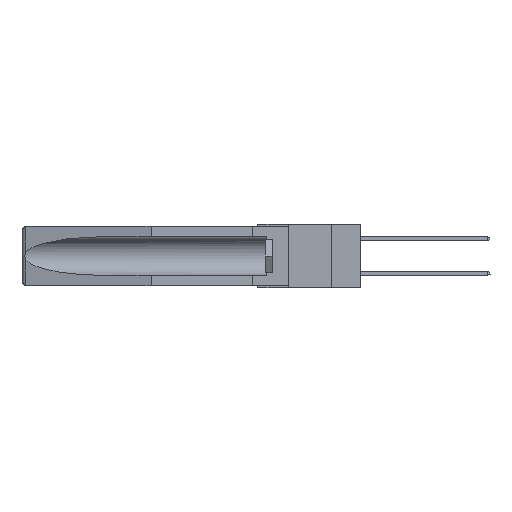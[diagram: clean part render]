
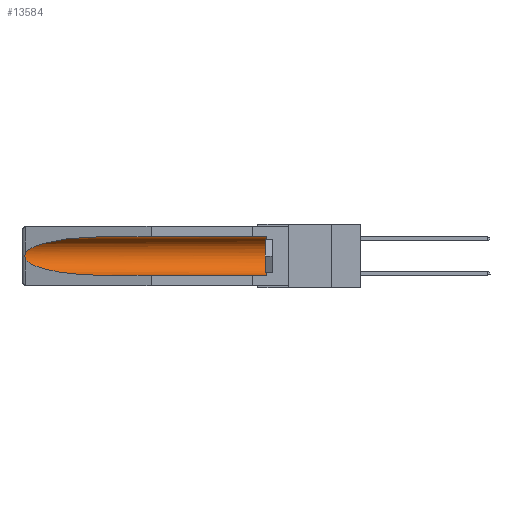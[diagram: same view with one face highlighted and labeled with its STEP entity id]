
A CAD part, left-side view. The second image highlights one B-rep face of the part: STEP entity #13584.
In plain terms, the highlighted cylindrical face has radius 2.857 mm (diameter 5.715 mm), a partial arc.
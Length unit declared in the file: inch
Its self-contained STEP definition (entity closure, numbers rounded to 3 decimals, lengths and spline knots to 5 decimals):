
#182 = CARTESIAN_POINT ( 'NONE',  ( 0.26537, 1.52718, -0.14972 ) ) ;
#677 =( BOUNDED_CURVE ( )  B_SPLINE_CURVE ( 3, ( #17258, #19397, #775, #2345 ),
 .UNSPECIFIED., .F., .F. ) 
 B_SPLINE_CURVE_WITH_KNOTS ( ( 4, 4 ),
 ( 0.1948, 1.5708 ),
 .UNSPECIFIED. ) 
 CURVE ( )  GEOMETRIC_REPRESENTATION_ITEM ( )  RATIONAL_B_SPLINE_CURVE ( ( 1., 0.848, 0.848, 1. ) ) 
 REPRESENTATION_ITEM ( '' )  );
#775 = CARTESIAN_POINT ( 'NONE',  ( 0.21114, 1.30732, -0.284 ) ) ;
#1628 = CARTESIAN_POINT ( 'NONE',  ( 0.25451, 1.48313, -0.09465 ) ) ;
#2092 = EDGE_CURVE ( 'NONE', #7967, #2964, #22281, .T. ) ;
#2345 = CARTESIAN_POINT ( 'NONE',  ( 0.155, 1.07973, -0.284 ) ) ;
#2677 = FACE_OUTER_BOUND ( 'NONE', #17705, .T. ) ;
#2744 = DIRECTION ( 'NONE',  ( 0., 1., 0. ) ) ;
#2804 = CARTESIAN_POINT ( 'NONE',  ( 0.26537, 1.52718, -0.19328 ) ) ;
#2964 = VERTEX_POINT ( 'NONE', #2804 ) ;
#3085 = AXIS2_PLACEMENT_3D ( 'NONE', #19926, #8956, #10681 ) ;
#3656 = CARTESIAN_POINT ( 'NONE',  ( 0.2673, 1.53269, -0.17917 ) ) ;
#3815 = CARTESIAN_POINT ( 'NONE',  ( 0.26654, 1.53092, -0.15636 ) ) ;
#3902 = CARTESIAN_POINT ( 'NONE',  ( 0.155, 1.07973, -0.059 ) ) ;
#3938 = EDGE_CURVE ( 'NONE', #17483, #12077, #10862, .T. ) ;
#4546 = CARTESIAN_POINT ( 'NONE',  ( 0.155, -0.30754, -0.059 ) ) ;
#6691 = VECTOR ( 'NONE', #20468, 39.37008 ) ;
#7471 = CARTESIAN_POINT ( 'NONE',  ( 0.155, -0.30754, -0.284 ) ) ;
#7504 = DIRECTION ( 'NONE',  ( 0., 0., 1. ) ) ;
#7678 = CYLINDRICAL_SURFACE ( 'NONE', #3085, 0.1125 ) ;
#7967 = VERTEX_POINT ( 'NONE', #19211 ) ;
#8046 = CARTESIAN_POINT ( 'NONE',  ( 0.155, 0.126, -0.059 ) ) ;
#8956 = DIRECTION ( 'NONE',  ( 0., 1., 0. ) ) ;
#9189 = CARTESIAN_POINT ( 'NONE',  ( 0.2675, 1.53308, -0.17534 ) ) ;
#9424 = VERTEX_POINT ( 'NONE', #3902 ) ;
#9440 = CARTESIAN_POINT ( 'NONE',  ( 0.26597, 1.5296, -0.19026 ) ) ;
#10066 = VERTEX_POINT ( 'NONE', #11141 ) ;
#10090 = EDGE_CURVE ( 'NONE', #17483, #10066, #21764, .T. ) ;
#10123 = ORIENTED_EDGE ( 'NONE', *, *, #10090, .F. ) ;
#10681 = DIRECTION ( 'NONE',  ( 0., 0., 1. ) ) ;
#10862 = CIRCLE ( 'NONE', #14207, 0.1125 ) ;
#11141 = CARTESIAN_POINT ( 'NONE',  ( 0.155, 1.07973, -0.284 ) ) ;
#12077 = VERTEX_POINT ( 'NONE', #8046 ) ;
#12626 = CARTESIAN_POINT ( 'NONE',  ( 0.155, 1.07973, -0.059 ) ) ;
#13039 = CARTESIAN_POINT ( 'NONE',  ( 0.2675, 1.53308, -0.16763 ) ) ;
#13059 = LINE ( 'NONE', #4546, #17134 ) ;
#13584 = ADVANCED_FACE ( 'NONE', ( #2677 ), #7678, .F. ) ;
#13747 =( BOUNDED_CURVE ( )  B_SPLINE_CURVE ( 3, ( #12626, #20155, #1628, #14687 ),
 .UNSPECIFIED., .F., .F. ) 
 B_SPLINE_CURVE_WITH_KNOTS ( ( 4, 4 ),
 ( 4.71239, 6.08839 ),
 .UNSPECIFIED. ) 
 CURVE ( )  GEOMETRIC_REPRESENTATION_ITEM ( )  RATIONAL_B_SPLINE_CURVE ( ( 1., 0.848, 0.848, 1. ) ) 
 REPRESENTATION_ITEM ( '' )  );
#14207 = AXIS2_PLACEMENT_3D ( 'NONE', #16804, #18644, #7504 ) ;
#14687 = CARTESIAN_POINT ( 'NONE',  ( 0.26537, 1.52718, -0.14972 ) ) ;
#15013 = CARTESIAN_POINT ( 'NONE',  ( 0.26597, 1.52961, -0.15275 ) ) ;
#15094 = ORIENTED_EDGE ( 'NONE', *, *, #3938, .T. ) ;
#15626 = CARTESIAN_POINT ( 'NONE',  ( 0.155, 0.126, -0.284 ) ) ;
#15882 = ORIENTED_EDGE ( 'NONE', *, *, #17510, .T. ) ;
#16804 = CARTESIAN_POINT ( 'NONE',  ( 0.155, 0.126, -0.1715 ) ) ;
#16865 = CARTESIAN_POINT ( 'NONE',  ( 0.2673, 1.5327, -0.16383 ) ) ;
#17092 = ORIENTED_EDGE ( 'NONE', *, *, #21011, .T. ) ;
#17134 = VECTOR ( 'NONE', #2744, 39.37008 ) ;
#17258 = CARTESIAN_POINT ( 'NONE',  ( 0.26537, 1.52718, -0.19328 ) ) ;
#17483 = VERTEX_POINT ( 'NONE', #15626 ) ;
#17510 = EDGE_CURVE ( 'NONE', #2964, #10066, #677, .T. ) ;
#17705 = EDGE_LOOP ( 'NONE', ( #17092, #23054, #15882, #10123, #15094, #21533 ) ) ;
#18644 = DIRECTION ( 'NONE',  ( 0., -1., 0. ) ) ;
#19211 = CARTESIAN_POINT ( 'NONE',  ( 0.26537, 1.52718, -0.14972 ) ) ;
#19397 = CARTESIAN_POINT ( 'NONE',  ( 0.25451, 1.48313, -0.24835 ) ) ;
#19926 = CARTESIAN_POINT ( 'NONE',  ( 0.155, -0.30754, -0.1715 ) ) ;
#20155 = CARTESIAN_POINT ( 'NONE',  ( 0.21114, 1.30732, -0.059 ) ) ;
#20468 = DIRECTION ( 'NONE',  ( 0., 1., 0. ) ) ;
#20869 = EDGE_CURVE ( 'NONE', #12077, #9424, #13059, .T. ) ;
#21011 = EDGE_CURVE ( 'NONE', #9424, #7967, #13747, .T. ) ;
#21533 = ORIENTED_EDGE ( 'NONE', *, *, #20869, .T. ) ;
#21764 = LINE ( 'NONE', #7471, #6691 ) ;
#22171 = CARTESIAN_POINT ( 'NONE',  ( 0.26537, 1.52718, -0.19328 ) ) ;
#22281 = B_SPLINE_CURVE_WITH_KNOTS ( 'NONE', 3,
 ( #182, #15013, #3815, #16865, #13039, #9189, #3656, #23915, #9440, #22171 ),
 .UNSPECIFIED., .F., .F.,
 ( 4, 2, 2, 2, 4 ),
 ( 0., 0.00029, 0.00058, 0.00087, 0.00117 ),
 .UNSPECIFIED. ) ;
#23054 = ORIENTED_EDGE ( 'NONE', *, *, #2092, .T. ) ;
#23915 = CARTESIAN_POINT ( 'NONE',  ( 0.26655, 1.53094, -0.18657 ) ) ;
